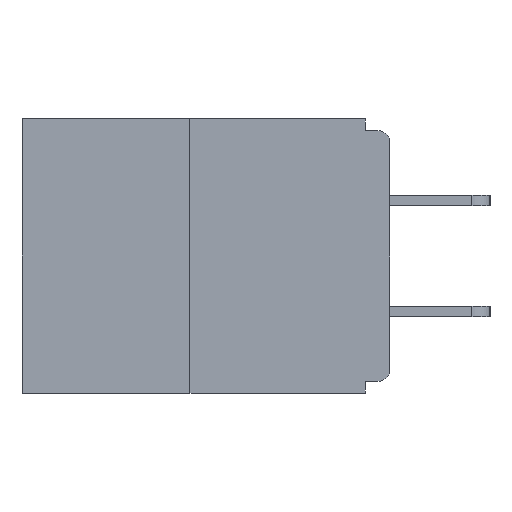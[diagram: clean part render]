
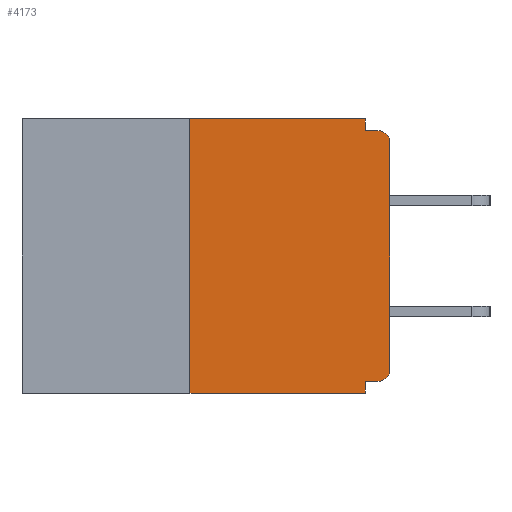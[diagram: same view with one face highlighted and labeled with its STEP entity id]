
A CAD part, left-side view. The second image highlights one B-rep face of the part: STEP entity #4173.
In plain terms, the highlighted planar face has unit normal (-1, 0, 0).
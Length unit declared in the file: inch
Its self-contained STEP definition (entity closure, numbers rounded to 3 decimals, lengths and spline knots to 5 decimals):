
#171 = EDGE_LOOP ( 'NONE', ( #17323, #7437, #2146, #14743, #18573, #5464, #13567, #17117, #18316, #8653 ) ) ;
#280 = DIRECTION ( 'NONE',  ( 0., -1., 0. ) ) ;
#866 = VECTOR ( 'NONE', #12791, 39.37008 ) ;
#878 = LINE ( 'NONE', #16121, #18642 ) ;
#1747 = LINE ( 'NONE', #7883, #866 ) ;
#1775 = VECTOR ( 'NONE', #14623, 39.37008 ) ;
#1863 = CARTESIAN_POINT ( 'NONE',  ( 0., 0.25, 0. ) ) ;
#2146 = ORIENTED_EDGE ( 'NONE', *, *, #15325, .T. ) ;
#2351 = EDGE_CURVE ( 'NONE', #5384, #9196, #1747, .T. ) ;
#2531 = CARTESIAN_POINT ( 'NONE',  ( 0., 0., -0.313 ) ) ;
#2745 = DIRECTION ( 'NONE',  ( 0., 0., -1. ) ) ;
#2847 = VERTEX_POINT ( 'NONE', #6858 ) ;
#3445 = EDGE_CURVE ( 'NONE', #5739, #11311, #9083, .T. ) ;
#3569 = VECTOR ( 'NONE', #280, 39.37008 ) ;
#3971 = CARTESIAN_POINT ( 'NONE',  ( 0., 0.015, -0.313 ) ) ;
#4173 = ADVANCED_FACE ( 'NONE', ( #4300 ), #7328, .F. ) ;
#4192 = DIRECTION ( 'NONE',  ( 0., 0., -1. ) ) ;
#4300 = FACE_OUTER_BOUND ( 'NONE', #171, .T. ) ;
#4430 = LINE ( 'NONE', #7768, #9508 ) ;
#5058 = VERTEX_POINT ( 'NONE', #7891 ) ;
#5384 = VERTEX_POINT ( 'NONE', #2531 ) ;
#5412 = CARTESIAN_POINT ( 'NONE',  ( 0., 0.46, 0. ) ) ;
#5464 = ORIENTED_EDGE ( 'NONE', *, *, #10655, .T. ) ;
#5684 = DIRECTION ( 'NONE',  ( -1., 0., 0. ) ) ;
#5739 = VERTEX_POINT ( 'NONE', #13363 ) ;
#6354 = CARTESIAN_POINT ( 'NONE',  ( 0., 0., -0.015 ) ) ;
#6432 = CIRCLE ( 'NONE', #11272, 0.015 ) ;
#6858 = CARTESIAN_POINT ( 'NONE',  ( 0., 0.25, -0.343 ) ) ;
#7328 = PLANE ( 'NONE',  #18829 ) ;
#7437 = ORIENTED_EDGE ( 'NONE', *, *, #16987, .F. ) ;
#7726 = CARTESIAN_POINT ( 'NONE',  ( 0., 0.46, 0. ) ) ;
#7768 = CARTESIAN_POINT ( 'NONE',  ( 0., 0.031, 0. ) ) ;
#7883 = CARTESIAN_POINT ( 'NONE',  ( 0., 0., 0. ) ) ;
#7891 = CARTESIAN_POINT ( 'NONE',  ( 0., 0.015, -0.328 ) ) ;
#8121 = CARTESIAN_POINT ( 'NONE',  ( 0., 0., -0.03 ) ) ;
#8155 = CARTESIAN_POINT ( 'NONE',  ( 0., 0.031, -0.343 ) ) ;
#8449 = VECTOR ( 'NONE', #18510, 39.37008 ) ;
#8653 = ORIENTED_EDGE ( 'NONE', *, *, #15934, .F. ) ;
#8810 = CARTESIAN_POINT ( 'NONE',  ( 0., 0.46, -0.343 ) ) ;
#8857 = DIRECTION ( 'NONE',  ( 1., 0., 0. ) ) ;
#9021 = CARTESIAN_POINT ( 'NONE',  ( 0., 0.25, 0. ) ) ;
#9083 = LINE ( 'NONE', #6354, #8449 ) ;
#9196 = VERTEX_POINT ( 'NONE', #8121 ) ;
#9384 = EDGE_CURVE ( 'NONE', #5058, #13215, #878, .T. ) ;
#9508 = VECTOR ( 'NONE', #2745, 39.37008 ) ;
#9768 = DIRECTION ( 'NONE',  ( 0., 0., -1. ) ) ;
#10415 = LINE ( 'NONE', #8810, #1775 ) ;
#10563 = LINE ( 'NONE', #15991, #13131 ) ;
#10655 = EDGE_CURVE ( 'NONE', #5058, #5384, #6432, .T. ) ;
#11202 = EDGE_CURVE ( 'NONE', #14673, #18879, #11236, .T. ) ;
#11236 = LINE ( 'NONE', #7726, #3569 ) ;
#11272 = AXIS2_PLACEMENT_3D ( 'NONE', #3971, #5684, #11637 ) ;
#11311 = VERTEX_POINT ( 'NONE', #14055 ) ;
#11449 = DIRECTION ( 'NONE',  ( 0., 1., 0. ) ) ;
#11464 = DIRECTION ( 'NONE',  ( -1., 0., 0. ) ) ;
#11637 = DIRECTION ( 'NONE',  ( 0., 0., -1. ) ) ;
#12719 = EDGE_CURVE ( 'NONE', #9196, #11311, #19641, .T. ) ;
#12791 = DIRECTION ( 'NONE',  ( 0., 0., 1. ) ) ;
#13131 = VECTOR ( 'NONE', #13560, 39.37008 ) ;
#13215 = VERTEX_POINT ( 'NONE', #19212 ) ;
#13363 = CARTESIAN_POINT ( 'NONE',  ( 0., 0.031, -0.015 ) ) ;
#13560 = DIRECTION ( 'NONE',  ( 0., 0., -1. ) ) ;
#13567 = ORIENTED_EDGE ( 'NONE', *, *, #2351, .T. ) ;
#13577 = EDGE_CURVE ( 'NONE', #13215, #16071, #10563, .T. ) ;
#14055 = CARTESIAN_POINT ( 'NONE',  ( 0., 0.015, -0.015 ) ) ;
#14623 = DIRECTION ( 'NONE',  ( 0., -1., 0. ) ) ;
#14673 = VERTEX_POINT ( 'NONE', #1863 ) ;
#14743 = ORIENTED_EDGE ( 'NONE', *, *, #13577, .F. ) ;
#15266 = VECTOR ( 'NONE', #19535, 39.37008 ) ;
#15325 = EDGE_CURVE ( 'NONE', #2847, #16071, #10415, .T. ) ;
#15934 = EDGE_CURVE ( 'NONE', #18879, #5739, #4430, .T. ) ;
#15991 = CARTESIAN_POINT ( 'NONE',  ( 0., 0.031, -0.343 ) ) ;
#16071 = VERTEX_POINT ( 'NONE', #8155 ) ;
#16121 = CARTESIAN_POINT ( 'NONE',  ( 0., 0., -0.328 ) ) ;
#16716 = LINE ( 'NONE', #9021, #15266 ) ;
#16738 = AXIS2_PLACEMENT_3D ( 'NONE', #17350, #11464, #9768 ) ;
#16987 = EDGE_CURVE ( 'NONE', #2847, #14673, #16716, .T. ) ;
#17117 = ORIENTED_EDGE ( 'NONE', *, *, #12719, .T. ) ;
#17323 = ORIENTED_EDGE ( 'NONE', *, *, #11202, .F. ) ;
#17350 = CARTESIAN_POINT ( 'NONE',  ( 0., 0.015, -0.03 ) ) ;
#18316 = ORIENTED_EDGE ( 'NONE', *, *, #3445, .F. ) ;
#18404 = CARTESIAN_POINT ( 'NONE',  ( 0., 0.031, 0. ) ) ;
#18510 = DIRECTION ( 'NONE',  ( 0., -1., 0. ) ) ;
#18573 = ORIENTED_EDGE ( 'NONE', *, *, #9384, .F. ) ;
#18642 = VECTOR ( 'NONE', #11449, 39.37008 ) ;
#18829 = AXIS2_PLACEMENT_3D ( 'NONE', #5412, #8857, #4192 ) ;
#18879 = VERTEX_POINT ( 'NONE', #18404 ) ;
#19212 = CARTESIAN_POINT ( 'NONE',  ( 0., 0.031, -0.328 ) ) ;
#19535 = DIRECTION ( 'NONE',  ( 0., 0., 1. ) ) ;
#19641 = CIRCLE ( 'NONE', #16738, 0.015 ) ;
